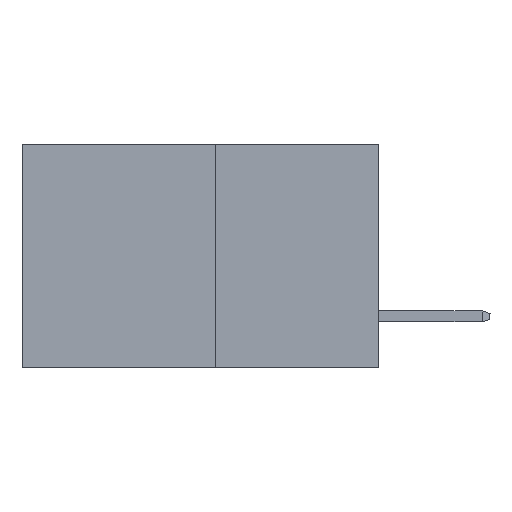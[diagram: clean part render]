
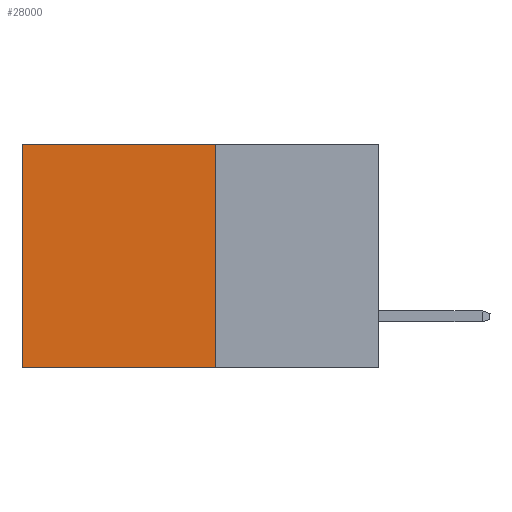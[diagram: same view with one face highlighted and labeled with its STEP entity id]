
A CAD part, left-side view. The second image highlights one B-rep face of the part: STEP entity #28000.
In plain terms, the highlighted planar face has unit normal (-1, 0, 0).
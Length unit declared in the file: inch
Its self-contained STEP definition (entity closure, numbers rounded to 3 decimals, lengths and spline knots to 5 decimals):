
#313 = CARTESIAN_POINT ( 'NONE',  ( 0.277, 0.27, 0. ) ) ;
#1082 = VECTOR ( 'NONE', #8773, 39.37008 ) ;
#2775 = PLANE ( 'NONE',  #11945 ) ;
#3121 = EDGE_CURVE ( 'NONE', #6294, #31358, #3415, .T. ) ;
#3415 = LINE ( 'NONE', #31493, #29723 ) ;
#3544 = CARTESIAN_POINT ( 'NONE',  ( 0.277, 0.27, 0. ) ) ;
#5903 = FACE_OUTER_BOUND ( 'NONE', #26471, .T. ) ;
#6294 = VERTEX_POINT ( 'NONE', #3544 ) ;
#6816 = CARTESIAN_POINT ( 'NONE',  ( 0.277, 0.59, -0.37 ) ) ;
#7307 = EDGE_CURVE ( 'NONE', #6294, #18467, #7930, .T. ) ;
#7930 = LINE ( 'NONE', #313, #1082 ) ;
#8773 = DIRECTION ( 'NONE',  ( 0., 1., 0. ) ) ;
#9390 = DIRECTION ( 'NONE',  ( 0., 0., -1. ) ) ;
#9594 = LINE ( 'NONE', #9888, #22286 ) ;
#9888 = CARTESIAN_POINT ( 'NONE',  ( 0.277, 0.27, -0.37 ) ) ;
#10648 = DIRECTION ( 'NONE',  ( 0., 0., -1. ) ) ;
#11945 = AXIS2_PLACEMENT_3D ( 'NONE', #23295, #25817, #10648 ) ;
#15362 = DIRECTION ( 'NONE',  ( 0., 0., -1. ) ) ;
#15513 = VECTOR ( 'NONE', #9390, 39.37008 ) ;
#17901 = ORIENTED_EDGE ( 'NONE', *, *, #23812, .F. ) ;
#18467 = VERTEX_POINT ( 'NONE', #21781 ) ;
#21781 = CARTESIAN_POINT ( 'NONE',  ( 0.277, 0.59, 0. ) ) ;
#22286 = VECTOR ( 'NONE', #30186, 39.37008 ) ;
#23295 = CARTESIAN_POINT ( 'NONE',  ( 0.277, 0.27, -0.37 ) ) ;
#23752 = LINE ( 'NONE', #6816, #15513 ) ;
#23812 = EDGE_CURVE ( 'NONE', #31358, #26155, #9594, .T. ) ;
#25379 = ORIENTED_EDGE ( 'NONE', *, *, #3121, .F. ) ;
#25817 = DIRECTION ( 'NONE',  ( 1., 0., 0. ) ) ;
#26155 = VERTEX_POINT ( 'NONE', #31182 ) ;
#26471 = EDGE_LOOP ( 'NONE', ( #29899, #17901, #25379, #29163 ) ) ;
#28000 = ADVANCED_FACE ( 'NONE', ( #5903 ), #2775, .F. ) ;
#28523 = EDGE_CURVE ( 'NONE', #18467, #26155, #23752, .T. ) ;
#29163 = ORIENTED_EDGE ( 'NONE', *, *, #7307, .T. ) ;
#29437 = CARTESIAN_POINT ( 'NONE',  ( 0.277, 0.27, -0.37 ) ) ;
#29723 = VECTOR ( 'NONE', #15362, 39.37008 ) ;
#29899 = ORIENTED_EDGE ( 'NONE', *, *, #28523, .T. ) ;
#30186 = DIRECTION ( 'NONE',  ( 0., 1., 0. ) ) ;
#31182 = CARTESIAN_POINT ( 'NONE',  ( 0.277, 0.59, -0.37 ) ) ;
#31358 = VERTEX_POINT ( 'NONE', #29437 ) ;
#31493 = CARTESIAN_POINT ( 'NONE',  ( 0.277, 0.27, -0.37 ) ) ;
